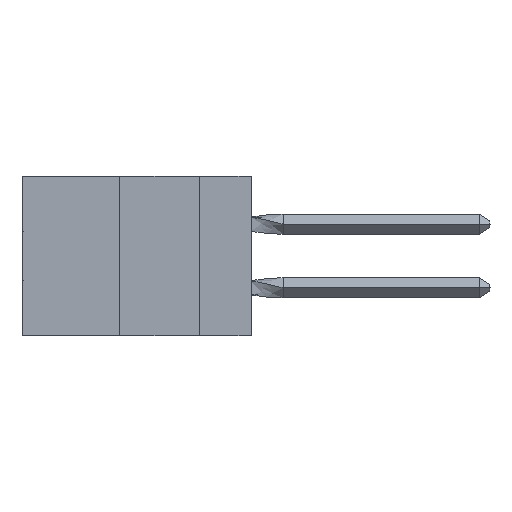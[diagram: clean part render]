
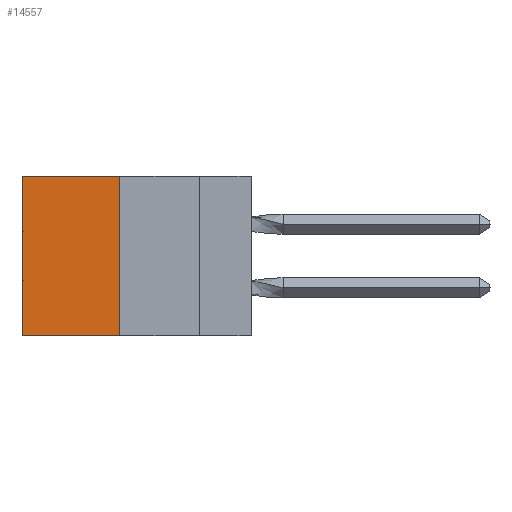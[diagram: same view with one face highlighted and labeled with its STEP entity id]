
A CAD part, left-side view. The second image highlights one B-rep face of the part: STEP entity #14557.
In plain terms, the highlighted planar face has unit normal (-1, 0, 0).
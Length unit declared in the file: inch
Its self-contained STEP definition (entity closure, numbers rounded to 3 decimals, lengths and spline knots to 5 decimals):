
#1845 = EDGE_CURVE ( 'NONE', #21825, #36004, #33276, .T. ) ;
#4446 = CARTESIAN_POINT ( 'NONE',  ( 0.305, 0.413, -0.5 ) ) ;
#5379 = DIRECTION ( 'NONE',  ( 0., 0., -1. ) ) ;
#6008 = CARTESIAN_POINT ( 'NONE',  ( 0.305, 0.72, -0.5 ) ) ;
#10323 = VECTOR ( 'NONE', #11435, 39.37008 ) ;
#11435 = DIRECTION ( 'NONE',  ( 0., 1., 0. ) ) ;
#14557 = ADVANCED_FACE ( 'NONE', ( #40908 ), #20909, .F. ) ;
#17105 = CARTESIAN_POINT ( 'NONE',  ( 0.305, 0.72, 0. ) ) ;
#17225 = CARTESIAN_POINT ( 'NONE',  ( 0.305, 0.413, 0. ) ) ;
#17500 = EDGE_CURVE ( 'NONE', #18986, #36004, #18118, .T. ) ;
#17721 = DIRECTION ( 'NONE',  ( 0., 0., -1. ) ) ;
#18034 = ORIENTED_EDGE ( 'NONE', *, *, #23576, .F. ) ;
#18118 = LINE ( 'NONE', #24704, #10323 ) ;
#18986 = VERTEX_POINT ( 'NONE', #34254 ) ;
#19169 = VECTOR ( 'NONE', #30183, 39.37008 ) ;
#19552 = CARTESIAN_POINT ( 'NONE',  ( 0.305, 0.413, -0.5 ) ) ;
#20909 = PLANE ( 'NONE',  #22852 ) ;
#21264 = CARTESIAN_POINT ( 'NONE',  ( 0.305, 0.413, 0. ) ) ;
#21825 = VERTEX_POINT ( 'NONE', #17105 ) ;
#22852 = AXIS2_PLACEMENT_3D ( 'NONE', #4446, #34796, #17721 ) ;
#23576 = EDGE_CURVE ( 'NONE', #41570, #18986, #32443, .T. ) ;
#24704 = CARTESIAN_POINT ( 'NONE',  ( 0.305, 0.413, -0.5 ) ) ;
#25873 = DIRECTION ( 'NONE',  ( 0., 0., -1. ) ) ;
#27313 = VECTOR ( 'NONE', #25873, 39.37008 ) ;
#30183 = DIRECTION ( 'NONE',  ( 0., 1., 0. ) ) ;
#31153 = ORIENTED_EDGE ( 'NONE', *, *, #1845, .T. ) ;
#32255 = VECTOR ( 'NONE', #5379, 39.37008 ) ;
#32443 = LINE ( 'NONE', #19552, #27313 ) ;
#32537 = LINE ( 'NONE', #17225, #19169 ) ;
#32893 = ORIENTED_EDGE ( 'NONE', *, *, #38064, .T. ) ;
#33276 = LINE ( 'NONE', #38497, #32255 ) ;
#34254 = CARTESIAN_POINT ( 'NONE',  ( 0.305, 0.413, -0.5 ) ) ;
#34796 = DIRECTION ( 'NONE',  ( 1., 0., 0. ) ) ;
#35600 = ORIENTED_EDGE ( 'NONE', *, *, #17500, .F. ) ;
#36004 = VERTEX_POINT ( 'NONE', #6008 ) ;
#37403 = EDGE_LOOP ( 'NONE', ( #31153, #35600, #18034, #32893 ) ) ;
#38064 = EDGE_CURVE ( 'NONE', #41570, #21825, #32537, .T. ) ;
#38497 = CARTESIAN_POINT ( 'NONE',  ( 0.305, 0.72, -0.5 ) ) ;
#40908 = FACE_OUTER_BOUND ( 'NONE', #37403, .T. ) ;
#41570 = VERTEX_POINT ( 'NONE', #21264 ) ;
